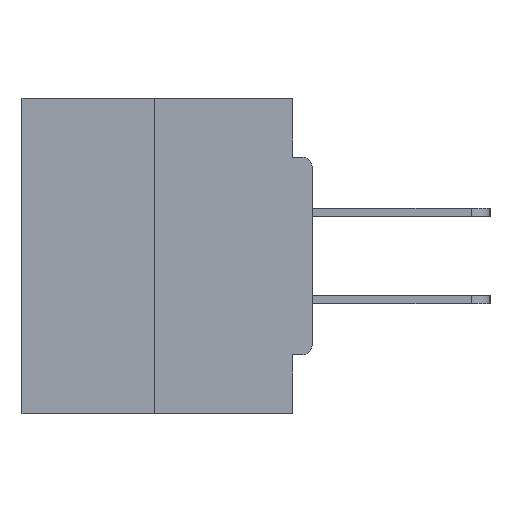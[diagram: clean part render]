
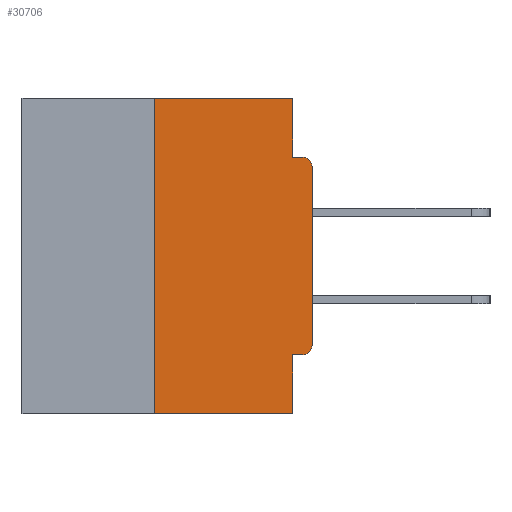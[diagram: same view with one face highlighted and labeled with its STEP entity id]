
A CAD part, left-side view. The second image highlights one B-rep face of the part: STEP entity #30706.
In plain terms, the highlighted planar face has unit normal (-1, 0, 0).
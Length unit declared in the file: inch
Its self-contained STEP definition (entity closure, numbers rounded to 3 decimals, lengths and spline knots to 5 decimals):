
#823 = CARTESIAN_POINT ( 'NONE',  ( 0., 0.015, -0.4065 ) ) ;
#1976 = CARTESIAN_POINT ( 'NONE',  ( 0., 0.031, -0.5 ) ) ;
#2024 = EDGE_CURVE ( 'NONE', #24462, #27191, #22420, .T. ) ;
#2557 = CARTESIAN_POINT ( 'NONE',  ( 0., 0.031, 0. ) ) ;
#2896 = DIRECTION ( 'NONE',  ( 0., 0., 1. ) ) ;
#3518 = ORIENTED_EDGE ( 'NONE', *, *, #26912, .F. ) ;
#3533 = LINE ( 'NONE', #11087, #10870 ) ;
#4438 = EDGE_LOOP ( 'NONE', ( #8655, #19263, #32303, #14810, #20422, #19338, #14122, #30641, #3518, #13319 ) ) ;
#4901 = CARTESIAN_POINT ( 'NONE',  ( 0., 0.25, 0. ) ) ;
#5018 = DIRECTION ( 'NONE',  ( 0., 0., 1. ) ) ;
#5312 = LINE ( 'NONE', #22865, #14136 ) ;
#5631 = EDGE_CURVE ( 'NONE', #27191, #7365, #23782, .T. ) ;
#5937 = DIRECTION ( 'NONE',  ( 0., 0., -1. ) ) ;
#6323 = CARTESIAN_POINT ( 'NONE',  ( 0., 0.031, -0.0935 ) ) ;
#7165 = DIRECTION ( 'NONE',  ( 0., 0., -1. ) ) ;
#7365 = VERTEX_POINT ( 'NONE', #13543 ) ;
#7464 = FACE_OUTER_BOUND ( 'NONE', #4438, .T. ) ;
#7930 = VERTEX_POINT ( 'NONE', #9724 ) ;
#7982 = CARTESIAN_POINT ( 'NONE',  ( 0., 0., -0.0935 ) ) ;
#8422 = EDGE_CURVE ( 'NONE', #7930, #24205, #12619, .T. ) ;
#8601 = CARTESIAN_POINT ( 'NONE',  ( 0., 0.031, -0.4065 ) ) ;
#8653 = VERTEX_POINT ( 'NONE', #1976 ) ;
#8655 = ORIENTED_EDGE ( 'NONE', *, *, #25561, .F. ) ;
#8799 = LINE ( 'NONE', #11414, #19007 ) ;
#8880 = VECTOR ( 'NONE', #5018, 39.37008 ) ;
#9026 = CARTESIAN_POINT ( 'NONE',  ( 0., 0.031, 0. ) ) ;
#9724 = CARTESIAN_POINT ( 'NONE',  ( 0., 0.25, -0.5 ) ) ;
#10249 = DIRECTION ( 'NONE',  ( 1., 0., 0. ) ) ;
#10626 = CARTESIAN_POINT ( 'NONE',  ( 0., 0.46, 0. ) ) ;
#10870 = VECTOR ( 'NONE', #21107, 39.37008 ) ;
#11003 = VECTOR ( 'NONE', #19873, 39.37008 ) ;
#11087 = CARTESIAN_POINT ( 'NONE',  ( 0., 0., -0.4065 ) ) ;
#11414 = CARTESIAN_POINT ( 'NONE',  ( 0., 0.031, -0.5 ) ) ;
#11828 = CARTESIAN_POINT ( 'NONE',  ( 0., 0.015, -0.1085 ) ) ;
#12426 = CARTESIAN_POINT ( 'NONE',  ( 0., 0.25, 0. ) ) ;
#12619 = LINE ( 'NONE', #4901, #16073 ) ;
#13319 = ORIENTED_EDGE ( 'NONE', *, *, #15584, .F. ) ;
#13329 = DIRECTION ( 'NONE',  ( -1., 0., 0. ) ) ;
#13543 = CARTESIAN_POINT ( 'NONE',  ( 0., 0.015, -0.0935 ) ) ;
#13563 = DIRECTION ( 'NONE',  ( 0., 0., -1. ) ) ;
#14122 = ORIENTED_EDGE ( 'NONE', *, *, #2024, .T. ) ;
#14136 = VECTOR ( 'NONE', #25187, 39.37008 ) ;
#14810 = ORIENTED_EDGE ( 'NONE', *, *, #31939, .F. ) ;
#14873 = PLANE ( 'NONE',  #15268 ) ;
#15264 = LINE ( 'NONE', #10626, #11003 ) ;
#15268 = AXIS2_PLACEMENT_3D ( 'NONE', #24881, #10249, #17177 ) ;
#15584 = EDGE_CURVE ( 'NONE', #30225, #16299, #32305, .T. ) ;
#16073 = VECTOR ( 'NONE', #2896, 39.37008 ) ;
#16299 = VERTEX_POINT ( 'NONE', #6323 ) ;
#16861 = VECTOR ( 'NONE', #20352, 39.37008 ) ;
#17177 = DIRECTION ( 'NONE',  ( 0., 0., -1. ) ) ;
#17244 = DIRECTION ( 'NONE',  ( -1., 0., 0. ) ) ;
#18066 = EDGE_CURVE ( 'NONE', #25378, #29130, #3533, .T. ) ;
#19007 = VECTOR ( 'NONE', #13563, 39.37008 ) ;
#19263 = ORIENTED_EDGE ( 'NONE', *, *, #8422, .F. ) ;
#19338 = ORIENTED_EDGE ( 'NONE', *, *, #32292, .T. ) ;
#19381 = VECTOR ( 'NONE', #7165, 39.37008 ) ;
#19873 = DIRECTION ( 'NONE',  ( 0., -1., 0. ) ) ;
#20352 = DIRECTION ( 'NONE',  ( 0., -1., 0. ) ) ;
#20422 = ORIENTED_EDGE ( 'NONE', *, *, #18066, .F. ) ;
#20867 = CARTESIAN_POINT ( 'NONE',  ( 0., 0.015, -0.3915 ) ) ;
#21107 = DIRECTION ( 'NONE',  ( 0., 1., 0. ) ) ;
#22420 = LINE ( 'NONE', #29965, #8880 ) ;
#22865 = CARTESIAN_POINT ( 'NONE',  ( 0., 0.46, -0.5 ) ) ;
#23782 = CIRCLE ( 'NONE', #27967, 0.015 ) ;
#24205 = VERTEX_POINT ( 'NONE', #12426 ) ;
#24445 = CARTESIAN_POINT ( 'NONE',  ( 0., 0., -0.1085 ) ) ;
#24462 = VERTEX_POINT ( 'NONE', #26362 ) ;
#24697 = EDGE_CURVE ( 'NONE', #7930, #8653, #5312, .T. ) ;
#24812 = LINE ( 'NONE', #7982, #16861 ) ;
#24881 = CARTESIAN_POINT ( 'NONE',  ( 0., 0.46, 0. ) ) ;
#25187 = DIRECTION ( 'NONE',  ( 0., -1., 0. ) ) ;
#25378 = VERTEX_POINT ( 'NONE', #823 ) ;
#25561 = EDGE_CURVE ( 'NONE', #24205, #30225, #15264, .T. ) ;
#26362 = CARTESIAN_POINT ( 'NONE',  ( 0., 0., -0.3915 ) ) ;
#26912 = EDGE_CURVE ( 'NONE', #16299, #7365, #24812, .T. ) ;
#27191 = VERTEX_POINT ( 'NONE', #24445 ) ;
#27967 = AXIS2_PLACEMENT_3D ( 'NONE', #11828, #17244, #29692 ) ;
#29130 = VERTEX_POINT ( 'NONE', #8601 ) ;
#29432 = CIRCLE ( 'NONE', #31546, 0.015 ) ;
#29692 = DIRECTION ( 'NONE',  ( 0., 0., -1. ) ) ;
#29965 = CARTESIAN_POINT ( 'NONE',  ( 0., 0., 0. ) ) ;
#30225 = VERTEX_POINT ( 'NONE', #9026 ) ;
#30641 = ORIENTED_EDGE ( 'NONE', *, *, #5631, .T. ) ;
#30706 = ADVANCED_FACE ( 'NONE', ( #7464 ), #14873, .F. ) ;
#31546 = AXIS2_PLACEMENT_3D ( 'NONE', #20867, #13329, #5937 ) ;
#31939 = EDGE_CURVE ( 'NONE', #29130, #8653, #8799, .T. ) ;
#32292 = EDGE_CURVE ( 'NONE', #25378, #24462, #29432, .T. ) ;
#32303 = ORIENTED_EDGE ( 'NONE', *, *, #24697, .T. ) ;
#32305 = LINE ( 'NONE', #2557, #19381 ) ;
